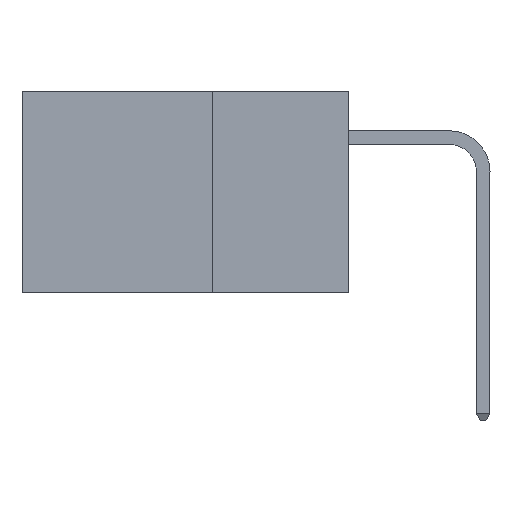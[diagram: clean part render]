
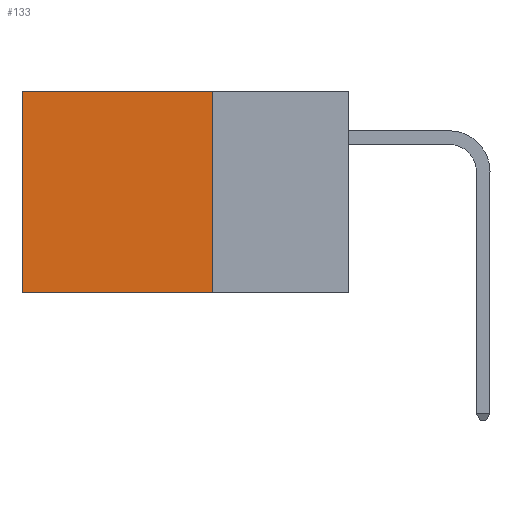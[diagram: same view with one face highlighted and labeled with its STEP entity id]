
A CAD part, left-side view. The second image highlights one B-rep face of the part: STEP entity #133.
In plain terms, the highlighted planar face has unit normal (-1, 0, 0).
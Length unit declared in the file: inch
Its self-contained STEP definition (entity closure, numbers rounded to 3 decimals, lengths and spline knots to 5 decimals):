
#127 = CARTESIAN_POINT ( 'NONE',  ( 0.2875, 0.6, 0. ) ) ;
#133 = ADVANCED_FACE ( 'NONE', ( #3833 ), #9917, .F. ) ;
#369 = LINE ( 'NONE', #4689, #8381 ) ;
#504 = VECTOR ( 'NONE', #1416, 39.37008 ) ;
#673 = EDGE_CURVE ( 'NONE', #767, #21220, #369, .T. ) ;
#767 = VERTEX_POINT ( 'NONE', #23361 ) ;
#1416 = DIRECTION ( 'NONE',  ( 0., 0., -1. ) ) ;
#3833 = FACE_OUTER_BOUND ( 'NONE', #22776, .T. ) ;
#4689 = CARTESIAN_POINT ( 'NONE',  ( 0.2875, 0.25, -0.37 ) ) ;
#4705 = DIRECTION ( 'NONE',  ( 0., 0., -1. ) ) ;
#7117 = AXIS2_PLACEMENT_3D ( 'NONE', #13344, #8142, #9997 ) ;
#8142 = DIRECTION ( 'NONE',  ( 1., 0., 0. ) ) ;
#8381 = VECTOR ( 'NONE', #20909, 39.37008 ) ;
#9012 = EDGE_CURVE ( 'NONE', #22139, #21220, #21412, .T. ) ;
#9077 = EDGE_CURVE ( 'NONE', #23417, #767, #19679, .T. ) ;
#9698 = VECTOR ( 'NONE', #14869, 39.37008 ) ;
#9917 = PLANE ( 'NONE',  #7117 ) ;
#9997 = DIRECTION ( 'NONE',  ( 0., 0., -1. ) ) ;
#11910 = EDGE_CURVE ( 'NONE', #23417, #22139, #14268, .T. ) ;
#12925 = ORIENTED_EDGE ( 'NONE', *, *, #11910, .T. ) ;
#13344 = CARTESIAN_POINT ( 'NONE',  ( 0.2875, 0.25, 0. ) ) ;
#13935 = CARTESIAN_POINT ( 'NONE',  ( 0.2875, 0.25, 0. ) ) ;
#14268 = LINE ( 'NONE', #18680, #9698 ) ;
#14688 = ORIENTED_EDGE ( 'NONE', *, *, #673, .F. ) ;
#14869 = DIRECTION ( 'NONE',  ( 0., 1., 0. ) ) ;
#15058 = VECTOR ( 'NONE', #4705, 39.37008 ) ;
#15522 = ORIENTED_EDGE ( 'NONE', *, *, #9077, .F. ) ;
#15606 = CARTESIAN_POINT ( 'NONE',  ( 0.2875, 0.6, 0. ) ) ;
#15720 = CARTESIAN_POINT ( 'NONE',  ( 0.2875, 0.6, -0.37 ) ) ;
#18680 = CARTESIAN_POINT ( 'NONE',  ( 0.2875, 0.25, 0. ) ) ;
#19679 = LINE ( 'NONE', #23303, #504 ) ;
#20909 = DIRECTION ( 'NONE',  ( 0., 1., 0. ) ) ;
#21220 = VERTEX_POINT ( 'NONE', #15720 ) ;
#21412 = LINE ( 'NONE', #15606, #15058 ) ;
#22139 = VERTEX_POINT ( 'NONE', #127 ) ;
#22776 = EDGE_LOOP ( 'NONE', ( #23163, #14688, #15522, #12925 ) ) ;
#23163 = ORIENTED_EDGE ( 'NONE', *, *, #9012, .T. ) ;
#23303 = CARTESIAN_POINT ( 'NONE',  ( 0.2875, 0.25, 0. ) ) ;
#23361 = CARTESIAN_POINT ( 'NONE',  ( 0.2875, 0.25, -0.37 ) ) ;
#23417 = VERTEX_POINT ( 'NONE', #13935 ) ;
